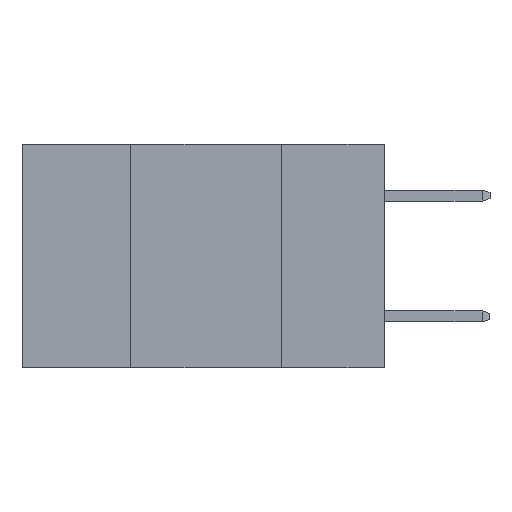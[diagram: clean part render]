
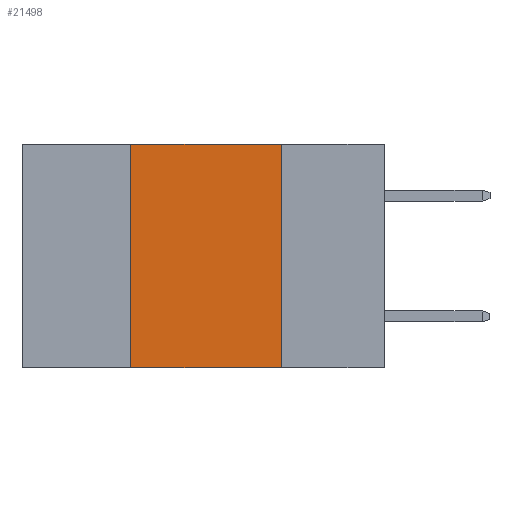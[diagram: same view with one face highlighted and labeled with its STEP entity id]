
A CAD part, left-side view. The second image highlights one B-rep face of the part: STEP entity #21498.
In plain terms, the highlighted planar face has unit normal (-1, 0, 0).
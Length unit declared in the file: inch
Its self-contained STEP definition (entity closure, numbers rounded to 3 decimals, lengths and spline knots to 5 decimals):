
#1662 = CARTESIAN_POINT ( 'NONE',  ( 0., 0.17, -0.37 ) ) ;
#2128 = LINE ( 'NONE', #20623, #21183 ) ;
#2916 = VERTEX_POINT ( 'NONE', #6776 ) ;
#3000 = LINE ( 'NONE', #17565, #12347 ) ;
#4581 = DIRECTION ( 'NONE',  ( 0., 0., -1. ) ) ;
#5253 = DIRECTION ( 'NONE',  ( 0., -1., 0. ) ) ;
#5787 = CARTESIAN_POINT ( 'NONE',  ( 0., 0.6, -0.37 ) ) ;
#6363 = PLANE ( 'NONE',  #21954 ) ;
#6578 = CARTESIAN_POINT ( 'NONE',  ( 0., 0.42, -0.37 ) ) ;
#6776 = CARTESIAN_POINT ( 'NONE',  ( 0., 0.42, 0. ) ) ;
#8212 = ORIENTED_EDGE ( 'NONE', *, *, #12886, .T. ) ;
#8455 = EDGE_CURVE ( 'NONE', #8536, #2916, #14465, .T. ) ;
#8536 = VERTEX_POINT ( 'NONE', #6578 ) ;
#10094 = DIRECTION ( 'NONE',  ( 0., -1., 0. ) ) ;
#10842 = ORIENTED_EDGE ( 'NONE', *, *, #16031, .F. ) ;
#11489 = DIRECTION ( 'NONE',  ( 0., 0., -1. ) ) ;
#11992 = CARTESIAN_POINT ( 'NONE',  ( 0., 0.6, 0. ) ) ;
#12347 = VECTOR ( 'NONE', #10094, 39.37008 ) ;
#12886 = EDGE_CURVE ( 'NONE', #8536, #20637, #23659, .T. ) ;
#14219 = VECTOR ( 'NONE', #5253, 39.37008 ) ;
#14465 = LINE ( 'NONE', #21742, #23352 ) ;
#14609 = CARTESIAN_POINT ( 'NONE',  ( 0., 0.17, 0. ) ) ;
#15820 = DIRECTION ( 'NONE',  ( 1., 0., 0. ) ) ;
#16031 = EDGE_CURVE ( 'NONE', #22388, #20637, #2128, .T. ) ;
#16215 = EDGE_CURVE ( 'NONE', #2916, #22388, #3000, .T. ) ;
#17045 = ORIENTED_EDGE ( 'NONE', *, *, #8455, .F. ) ;
#17565 = CARTESIAN_POINT ( 'NONE',  ( 0., 0.6, 0. ) ) ;
#20623 = CARTESIAN_POINT ( 'NONE',  ( 0., 0.17, 0. ) ) ;
#20637 = VERTEX_POINT ( 'NONE', #1662 ) ;
#21153 = ORIENTED_EDGE ( 'NONE', *, *, #16215, .F. ) ;
#21183 = VECTOR ( 'NONE', #11489, 39.37008 ) ;
#21498 = ADVANCED_FACE ( 'NONE', ( #21757 ), #6363, .F. ) ;
#21742 = CARTESIAN_POINT ( 'NONE',  ( 0., 0.42, 0. ) ) ;
#21757 = FACE_OUTER_BOUND ( 'NONE', #22845, .T. ) ;
#21954 = AXIS2_PLACEMENT_3D ( 'NONE', #11992, #15820, #4581 ) ;
#22326 = DIRECTION ( 'NONE',  ( 0., 0., 1. ) ) ;
#22388 = VERTEX_POINT ( 'NONE', #14609 ) ;
#22845 = EDGE_LOOP ( 'NONE', ( #10842, #21153, #17045, #8212 ) ) ;
#23352 = VECTOR ( 'NONE', #22326, 39.37008 ) ;
#23659 = LINE ( 'NONE', #5787, #14219 ) ;
